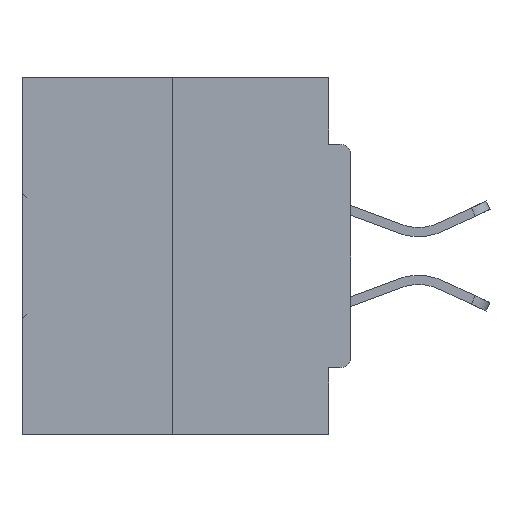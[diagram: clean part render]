
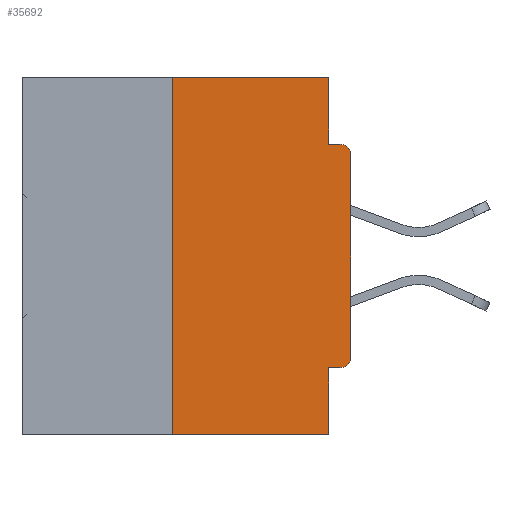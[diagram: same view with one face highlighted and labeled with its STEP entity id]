
A CAD part, left-side view. The second image highlights one B-rep face of the part: STEP entity #35692.
In plain terms, the highlighted planar face has unit normal (-1, 0, 0).
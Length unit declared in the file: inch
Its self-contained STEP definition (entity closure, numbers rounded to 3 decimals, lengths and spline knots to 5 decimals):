
#201 = VECTOR ( 'NONE', #2425, 39.37008 ) ;
#778 = CARTESIAN_POINT ( 'NONE',  ( 0., 0.031, -0.4065 ) ) ;
#787 = EDGE_CURVE ( 'NONE', #33036, #5164, #29142, .T. ) ;
#1737 = VERTEX_POINT ( 'NONE', #37863 ) ;
#2425 = DIRECTION ( 'NONE',  ( 0., 1., 0. ) ) ;
#3698 = CARTESIAN_POINT ( 'NONE',  ( 0., 0.031, -0.5 ) ) ;
#3778 = CARTESIAN_POINT ( 'NONE',  ( 0., 0.46, 0. ) ) ;
#5164 = VERTEX_POINT ( 'NONE', #19804 ) ;
#5713 = VECTOR ( 'NONE', #40195, 39.37008 ) ;
#8174 = VECTOR ( 'NONE', #14399, 39.37008 ) ;
#8685 = LINE ( 'NONE', #22206, #14267 ) ;
#8865 = LINE ( 'NONE', #3778, #44959 ) ;
#9413 = DIRECTION ( 'NONE',  ( 0., 0., -1. ) ) ;
#10083 = CARTESIAN_POINT ( 'NONE',  ( 0., 0.46, -0.5 ) ) ;
#10357 = EDGE_CURVE ( 'NONE', #42397, #1737, #20616, .T. ) ;
#10623 = AXIS2_PLACEMENT_3D ( 'NONE', #37194, #19504, #33756 ) ;
#11294 = LINE ( 'NONE', #11911, #5713 ) ;
#11911 = CARTESIAN_POINT ( 'NONE',  ( 0., 0.031, 0. ) ) ;
#12033 = ORIENTED_EDGE ( 'NONE', *, *, #787, .F. ) ;
#12397 = DIRECTION ( 'NONE',  ( -1., 0., 0. ) ) ;
#12955 = CARTESIAN_POINT ( 'NONE',  ( 0., 0.25, 0. ) ) ;
#14267 = VECTOR ( 'NONE', #25470, 39.37008 ) ;
#14372 = ORIENTED_EDGE ( 'NONE', *, *, #33661, .F. ) ;
#14399 = DIRECTION ( 'NONE',  ( 0., 0., -1. ) ) ;
#17036 = LINE ( 'NONE', #10083, #24842 ) ;
#18405 = EDGE_LOOP ( 'NONE', ( #45016, #12033, #40886, #27801, #14372, #34205, #44565, #28148, #19143, #31433 ) ) ;
#19143 = ORIENTED_EDGE ( 'NONE', *, *, #10357, .F. ) ;
#19504 = DIRECTION ( 'NONE',  ( 1., 0., 0. ) ) ;
#19804 = CARTESIAN_POINT ( 'NONE',  ( 0., 0.25, 0. ) ) ;
#19991 = CARTESIAN_POINT ( 'NONE',  ( 0., 0., -0.4065 ) ) ;
#20616 = LINE ( 'NONE', #38124, #21200 ) ;
#20718 = EDGE_CURVE ( 'NONE', #33430, #22216, #32066, .T. ) ;
#20804 = VECTOR ( 'NONE', #44761, 39.37008 ) ;
#21200 = VECTOR ( 'NONE', #34993, 39.37008 ) ;
#22206 = CARTESIAN_POINT ( 'NONE',  ( 0., 0., 0. ) ) ;
#22216 = VERTEX_POINT ( 'NONE', #33512 ) ;
#23467 = CARTESIAN_POINT ( 'NONE',  ( 0., 0.25, -0.5 ) ) ;
#24842 = VECTOR ( 'NONE', #38679, 39.37008 ) ;
#25310 = VERTEX_POINT ( 'NONE', #29842 ) ;
#25470 = DIRECTION ( 'NONE',  ( 0., 0., 1. ) ) ;
#26289 = LINE ( 'NONE', #19991, #201 ) ;
#26321 = AXIS2_PLACEMENT_3D ( 'NONE', #44066, #12397, #40392 ) ;
#27501 = CARTESIAN_POINT ( 'NONE',  ( 0., 0.031, 0. ) ) ;
#27801 = ORIENTED_EDGE ( 'NONE', *, *, #20718, .F. ) ;
#28148 = ORIENTED_EDGE ( 'NONE', *, *, #45823, .T. ) ;
#28176 = DIRECTION ( 'NONE',  ( 0., -1., 0. ) ) ;
#29142 = LINE ( 'NONE', #12955, #20804 ) ;
#29698 = CARTESIAN_POINT ( 'NONE',  ( 0., 0.015, -0.4065 ) ) ;
#29842 = CARTESIAN_POINT ( 'NONE',  ( 0., 0., -0.3915 ) ) ;
#30052 = PLANE ( 'NONE',  #10623 ) ;
#31433 = ORIENTED_EDGE ( 'NONE', *, *, #33599, .F. ) ;
#32018 = CARTESIAN_POINT ( 'NONE',  ( 0., 0.031, -0.0935 ) ) ;
#32066 = LINE ( 'NONE', #3698, #8174 ) ;
#32863 = AXIS2_PLACEMENT_3D ( 'NONE', #37369, #44776, #9413 ) ;
#33036 = VERTEX_POINT ( 'NONE', #23467 ) ;
#33091 = VERTEX_POINT ( 'NONE', #44976 ) ;
#33430 = VERTEX_POINT ( 'NONE', #778 ) ;
#33512 = CARTESIAN_POINT ( 'NONE',  ( 0., 0.031, -0.5 ) ) ;
#33599 = EDGE_CURVE ( 'NONE', #44151, #42397, #11294, .T. ) ;
#33661 = EDGE_CURVE ( 'NONE', #40709, #33430, #26289, .T. ) ;
#33675 = EDGE_CURVE ( 'NONE', #40709, #25310, #36289, .T. ) ;
#33756 = DIRECTION ( 'NONE',  ( 0., 0., -1. ) ) ;
#34205 = ORIENTED_EDGE ( 'NONE', *, *, #33675, .T. ) ;
#34993 = DIRECTION ( 'NONE',  ( 0., -1., 0. ) ) ;
#35525 = FACE_OUTER_BOUND ( 'NONE', #18405, .T. ) ;
#35692 = ADVANCED_FACE ( 'NONE', ( #35525 ), #30052, .F. ) ;
#36289 = CIRCLE ( 'NONE', #32863, 0.015 ) ;
#37194 = CARTESIAN_POINT ( 'NONE',  ( 0., 0.46, 0. ) ) ;
#37369 = CARTESIAN_POINT ( 'NONE',  ( 0., 0.015, -0.3915 ) ) ;
#37863 = CARTESIAN_POINT ( 'NONE',  ( 0., 0.015, -0.0935 ) ) ;
#38124 = CARTESIAN_POINT ( 'NONE',  ( 0., 0., -0.0935 ) ) ;
#38679 = DIRECTION ( 'NONE',  ( 0., -1., 0. ) ) ;
#39331 = EDGE_CURVE ( 'NONE', #5164, #44151, #8865, .T. ) ;
#40195 = DIRECTION ( 'NONE',  ( 0., 0., -1. ) ) ;
#40392 = DIRECTION ( 'NONE',  ( 0., 0., -1. ) ) ;
#40709 = VERTEX_POINT ( 'NONE', #29698 ) ;
#40886 = ORIENTED_EDGE ( 'NONE', *, *, #41099, .T. ) ;
#41099 = EDGE_CURVE ( 'NONE', #33036, #22216, #17036, .T. ) ;
#41336 = EDGE_CURVE ( 'NONE', #25310, #33091, #8685, .T. ) ;
#41515 = CIRCLE ( 'NONE', #26321, 0.015 ) ;
#42397 = VERTEX_POINT ( 'NONE', #32018 ) ;
#44066 = CARTESIAN_POINT ( 'NONE',  ( 0., 0.015, -0.1085 ) ) ;
#44151 = VERTEX_POINT ( 'NONE', #27501 ) ;
#44565 = ORIENTED_EDGE ( 'NONE', *, *, #41336, .T. ) ;
#44761 = DIRECTION ( 'NONE',  ( 0., 0., 1. ) ) ;
#44776 = DIRECTION ( 'NONE',  ( -1., 0., 0. ) ) ;
#44959 = VECTOR ( 'NONE', #28176, 39.37008 ) ;
#44976 = CARTESIAN_POINT ( 'NONE',  ( 0., 0., -0.1085 ) ) ;
#45016 = ORIENTED_EDGE ( 'NONE', *, *, #39331, .F. ) ;
#45823 = EDGE_CURVE ( 'NONE', #33091, #1737, #41515, .T. ) ;
